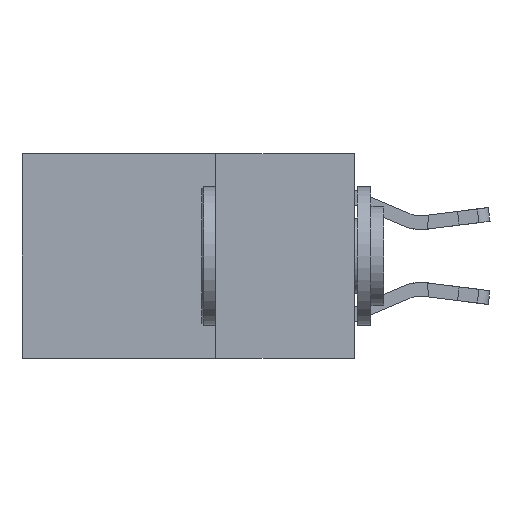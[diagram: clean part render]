
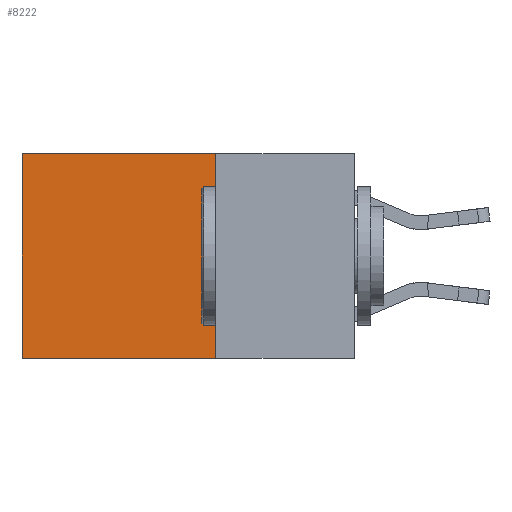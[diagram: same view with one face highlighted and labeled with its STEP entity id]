
A CAD part, left-side view. The second image highlights one B-rep face of the part: STEP entity #8222.
In plain terms, the highlighted planar face has unit normal (-1, 0, 0).
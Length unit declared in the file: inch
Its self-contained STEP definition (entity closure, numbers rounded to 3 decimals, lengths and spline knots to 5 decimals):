
#133 = CARTESIAN_POINT ( 'NONE',  ( 0.2625, 0.25, 0. ) ) ;
#139 = CARTESIAN_POINT ( 'NONE',  ( 0.2625, 0.25, -0.37 ) ) ;
#733 = LINE ( 'NONE', #133, #9123 ) ;
#837 = ORIENTED_EDGE ( 'NONE', *, *, #6851, .F. ) ;
#2211 = LINE ( 'NONE', #12994, #17402 ) ;
#2614 = EDGE_CURVE ( 'NONE', #11784, #2631, #7507, .T. ) ;
#2631 = VERTEX_POINT ( 'NONE', #9492 ) ;
#3049 = DIRECTION ( 'NONE',  ( 1., 0., 0. ) ) ;
#5110 = DIRECTION ( 'NONE',  ( 0., 1., 0. ) ) ;
#5129 = CARTESIAN_POINT ( 'NONE',  ( 0.2625, 0.6, 0. ) ) ;
#6033 = CARTESIAN_POINT ( 'NONE',  ( 0.2625, 0.25, 0. ) ) ;
#6596 = EDGE_CURVE ( 'NONE', #11110, #2631, #14207, .T. ) ;
#6851 = EDGE_CURVE ( 'NONE', #8783, #11784, #2211, .T. ) ;
#7172 = DIRECTION ( 'NONE',  ( 0., 0., -1. ) ) ;
#7507 = LINE ( 'NONE', #15367, #18673 ) ;
#8222 = ADVANCED_FACE ( 'NONE', ( #16898 ), #10446, .F. ) ;
#8289 = EDGE_CURVE ( 'NONE', #8783, #11110, #733, .T. ) ;
#8783 = VERTEX_POINT ( 'NONE', #13154 ) ;
#9123 = VECTOR ( 'NONE', #13498, 39.37008 ) ;
#9492 = CARTESIAN_POINT ( 'NONE',  ( 0.2625, 0.6, -0.37 ) ) ;
#10446 = PLANE ( 'NONE',  #12320 ) ;
#10814 = VECTOR ( 'NONE', #13900, 39.37008 ) ;
#11110 = VERTEX_POINT ( 'NONE', #18362 ) ;
#11784 = VERTEX_POINT ( 'NONE', #139 ) ;
#12067 = ORIENTED_EDGE ( 'NONE', *, *, #2614, .F. ) ;
#12320 = AXIS2_PLACEMENT_3D ( 'NONE', #6033, #3049, #13370 ) ;
#12791 = ORIENTED_EDGE ( 'NONE', *, *, #6596, .T. ) ;
#12994 = CARTESIAN_POINT ( 'NONE',  ( 0.2625, 0.25, 0. ) ) ;
#13154 = CARTESIAN_POINT ( 'NONE',  ( 0.2625, 0.25, 0. ) ) ;
#13370 = DIRECTION ( 'NONE',  ( 0., 0., -1. ) ) ;
#13498 = DIRECTION ( 'NONE',  ( 0., 1., 0. ) ) ;
#13900 = DIRECTION ( 'NONE',  ( 0., 0., -1. ) ) ;
#14207 = LINE ( 'NONE', #5129, #10814 ) ;
#15367 = CARTESIAN_POINT ( 'NONE',  ( 0.2625, 0.25, -0.37 ) ) ;
#16140 = EDGE_LOOP ( 'NONE', ( #12791, #12067, #837, #18554 ) ) ;
#16898 = FACE_OUTER_BOUND ( 'NONE', #16140, .T. ) ;
#17402 = VECTOR ( 'NONE', #7172, 39.37008 ) ;
#18362 = CARTESIAN_POINT ( 'NONE',  ( 0.2625, 0.6, 0. ) ) ;
#18554 = ORIENTED_EDGE ( 'NONE', *, *, #8289, .T. ) ;
#18673 = VECTOR ( 'NONE', #5110, 39.37008 ) ;
